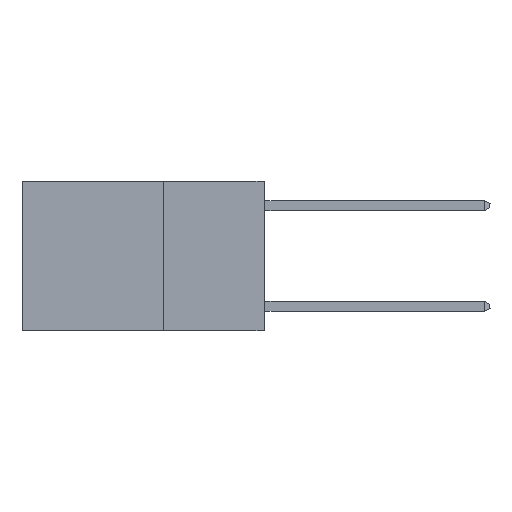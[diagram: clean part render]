
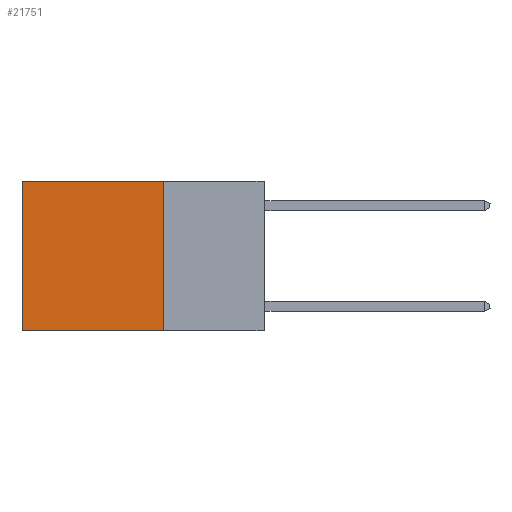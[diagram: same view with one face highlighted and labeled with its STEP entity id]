
A CAD part, left-side view. The second image highlights one B-rep face of the part: STEP entity #21751.
In plain terms, the highlighted planar face has unit normal (-1, 0, 0).
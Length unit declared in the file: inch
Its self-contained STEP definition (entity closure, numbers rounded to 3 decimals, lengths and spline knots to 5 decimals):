
#128 = VECTOR ( 'NONE', #13118, 39.37008 ) ;
#704 = VERTEX_POINT ( 'NONE', #20193 ) ;
#2269 = PLANE ( 'NONE',  #17262 ) ;
#2497 = FACE_OUTER_BOUND ( 'NONE', #23327, .T. ) ;
#2978 = EDGE_CURVE ( 'NONE', #704, #3836, #11341, .T. ) ;
#3144 = VECTOR ( 'NONE', #22461, 39.37008 ) ;
#3836 = VERTEX_POINT ( 'NONE', #14804 ) ;
#5734 = CARTESIAN_POINT ( 'NONE',  ( 0.2625, 0.6, 0. ) ) ;
#5884 = LINE ( 'NONE', #11149, #6009 ) ;
#6009 = VECTOR ( 'NONE', #20141, 39.37008 ) ;
#7659 = EDGE_CURVE ( 'NONE', #7861, #9662, #5884, .T. ) ;
#7861 = VERTEX_POINT ( 'NONE', #19411 ) ;
#8510 = EDGE_CURVE ( 'NONE', #704, #7861, #10704, .T. ) ;
#9513 = DIRECTION ( 'NONE',  ( 0., 0., -1. ) ) ;
#9662 = VERTEX_POINT ( 'NONE', #19041 ) ;
#10704 = LINE ( 'NONE', #21608, #13634 ) ;
#11149 = CARTESIAN_POINT ( 'NONE',  ( 0.2625, 0.25, -0.37 ) ) ;
#11341 = LINE ( 'NONE', #13114, #3144 ) ;
#11430 = CARTESIAN_POINT ( 'NONE',  ( 0.2625, 0.25, 0. ) ) ;
#12602 = DIRECTION ( 'NONE',  ( 0., 0., -1. ) ) ;
#13114 = CARTESIAN_POINT ( 'NONE',  ( 0.2625, 0.25, 0. ) ) ;
#13118 = DIRECTION ( 'NONE',  ( 0., 0., -1. ) ) ;
#13323 = DIRECTION ( 'NONE',  ( 1., 0., 0. ) ) ;
#13634 = VECTOR ( 'NONE', #12602, 39.37008 ) ;
#14804 = CARTESIAN_POINT ( 'NONE',  ( 0.2625, 0.6, 0. ) ) ;
#15751 = ORIENTED_EDGE ( 'NONE', *, *, #2978, .T. ) ;
#16661 = LINE ( 'NONE', #5734, #128 ) ;
#17161 = ORIENTED_EDGE ( 'NONE', *, *, #8510, .F. ) ;
#17262 = AXIS2_PLACEMENT_3D ( 'NONE', #11430, #13323, #9513 ) ;
#18449 = ORIENTED_EDGE ( 'NONE', *, *, #19268, .T. ) ;
#19041 = CARTESIAN_POINT ( 'NONE',  ( 0.2625, 0.6, -0.37 ) ) ;
#19268 = EDGE_CURVE ( 'NONE', #3836, #9662, #16661, .T. ) ;
#19411 = CARTESIAN_POINT ( 'NONE',  ( 0.2625, 0.25, -0.37 ) ) ;
#20141 = DIRECTION ( 'NONE',  ( 0., 1., 0. ) ) ;
#20193 = CARTESIAN_POINT ( 'NONE',  ( 0.2625, 0.25, 0. ) ) ;
#21608 = CARTESIAN_POINT ( 'NONE',  ( 0.2625, 0.25, 0. ) ) ;
#21751 = ADVANCED_FACE ( 'NONE', ( #2497 ), #2269, .F. ) ;
#21920 = ORIENTED_EDGE ( 'NONE', *, *, #7659, .F. ) ;
#22461 = DIRECTION ( 'NONE',  ( 0., 1., 0. ) ) ;
#23327 = EDGE_LOOP ( 'NONE', ( #18449, #21920, #17161, #15751 ) ) ;
